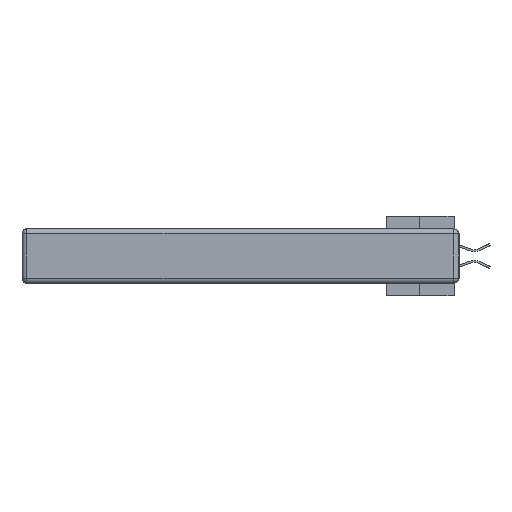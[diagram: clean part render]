
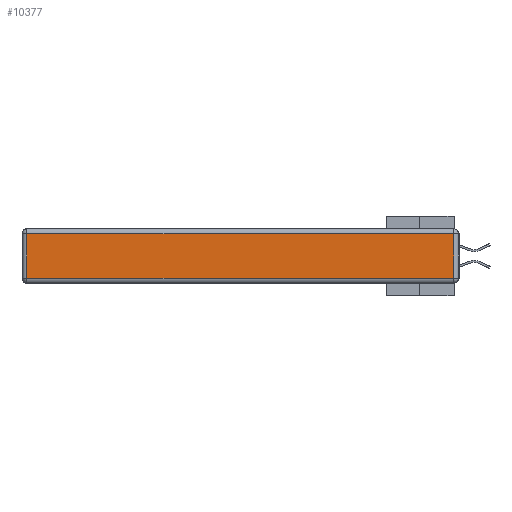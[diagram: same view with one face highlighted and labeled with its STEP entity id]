
A CAD part, left-side view. The second image highlights one B-rep face of the part: STEP entity #10377.
In plain terms, the highlighted planar face has unit normal (-1, 0, 0).
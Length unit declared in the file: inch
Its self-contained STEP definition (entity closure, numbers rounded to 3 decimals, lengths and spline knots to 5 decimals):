
#1856 = EDGE_CURVE ( 'NONE', #29596, #5960, #6606, .T. ) ;
#2635 = ORIENTED_EDGE ( 'NONE', *, *, #25769, .T. ) ;
#3196 = VECTOR ( 'NONE', #14924, 39.37008 ) ;
#4102 = LINE ( 'NONE', #23390, #7532 ) ;
#4116 = LINE ( 'NONE', #6034, #14034 ) ;
#5839 = CARTESIAN_POINT ( 'NONE',  ( 0., 2.72, -0.03 ) ) ;
#5960 = VERTEX_POINT ( 'NONE', #27580 ) ;
#6034 = CARTESIAN_POINT ( 'NONE',  ( 0., 0.03, -0.343 ) ) ;
#6606 = LINE ( 'NONE', #9155, #3196 ) ;
#7532 = VECTOR ( 'NONE', #29368, 39.37008 ) ;
#8804 = CARTESIAN_POINT ( 'NONE',  ( 0., 0.03, -0.03 ) ) ;
#9155 = CARTESIAN_POINT ( 'NONE',  ( 0., 0., -0.313 ) ) ;
#10377 = ADVANCED_FACE ( 'NONE', ( #31568 ), #33262, .T. ) ;
#10533 = DIRECTION ( 'NONE',  ( 0., 1., 0. ) ) ;
#10810 = ORIENTED_EDGE ( 'NONE', *, *, #12494, .T. ) ;
#11360 = DIRECTION ( 'NONE',  ( 0., 0., 1. ) ) ;
#11706 = EDGE_CURVE ( 'NONE', #17650, #34321, #16640, .T. ) ;
#12494 = EDGE_CURVE ( 'NONE', #34321, #29596, #4102, .T. ) ;
#13309 = CARTESIAN_POINT ( 'NONE',  ( 0., 2.72, -0.313 ) ) ;
#13590 = AXIS2_PLACEMENT_3D ( 'NONE', #33149, #16558, #35932 ) ;
#14034 = VECTOR ( 'NONE', #11360, 39.37008 ) ;
#14924 = DIRECTION ( 'NONE',  ( 0., -1., 0. ) ) ;
#16558 = DIRECTION ( 'NONE',  ( -1., 0., 0. ) ) ;
#16640 = LINE ( 'NONE', #30284, #27949 ) ;
#17650 = VERTEX_POINT ( 'NONE', #8804 ) ;
#18659 = ORIENTED_EDGE ( 'NONE', *, *, #11706, .T. ) ;
#23063 = EDGE_LOOP ( 'NONE', ( #25822, #2635, #18659, #10810 ) ) ;
#23390 = CARTESIAN_POINT ( 'NONE',  ( 0., 2.72, -0.343 ) ) ;
#25769 = EDGE_CURVE ( 'NONE', #5960, #17650, #4116, .T. ) ;
#25822 = ORIENTED_EDGE ( 'NONE', *, *, #1856, .T. ) ;
#27580 = CARTESIAN_POINT ( 'NONE',  ( 0., 0.03, -0.313 ) ) ;
#27949 = VECTOR ( 'NONE', #10533, 39.37008 ) ;
#29368 = DIRECTION ( 'NONE',  ( 0., 0., -1. ) ) ;
#29596 = VERTEX_POINT ( 'NONE', #13309 ) ;
#30284 = CARTESIAN_POINT ( 'NONE',  ( 0., 2.75, -0.03 ) ) ;
#31568 = FACE_OUTER_BOUND ( 'NONE', #23063, .T. ) ;
#33149 = CARTESIAN_POINT ( 'NONE',  ( 0., 0., -0.343 ) ) ;
#33262 = PLANE ( 'NONE',  #13590 ) ;
#34321 = VERTEX_POINT ( 'NONE', #5839 ) ;
#35932 = DIRECTION ( 'NONE',  ( 0., 0., 1. ) ) ;
